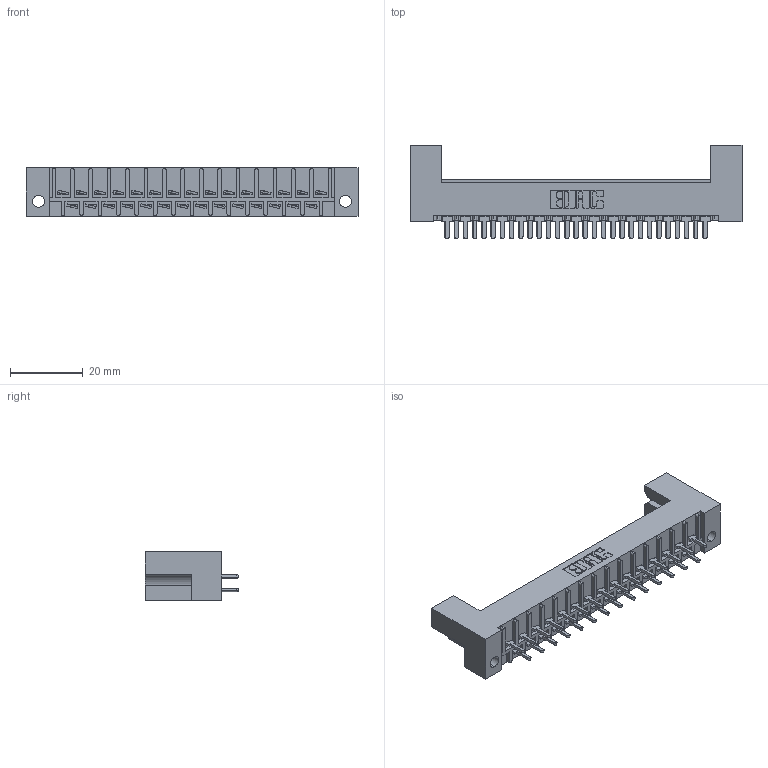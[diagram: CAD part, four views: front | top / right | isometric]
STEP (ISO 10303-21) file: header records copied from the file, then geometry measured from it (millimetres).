
FILE_DESCRIPTION (( 'STEP AP203' ), '1' );
FILE_NAME ('408-029-525-222.STEP', '2019-11-04T19:03:35', ( '' ), ( '' ), 'SwSTEP 2.0', 'SolidWorks 2016', '' );
FILE_SCHEMA (( 'CONFIG_CONTROL_DESIGN' ));
Length unit declared in the file: inch
Products named in the file (4): 408 Part_029 - 2; 408-029-525-222; 408-290-001_408-290-125 - Bottom; 408-290-001_408-290-125 - Top
Assembly tree (30 placements, depth 2):
  408-029-525-222
    408 Part_029 - 2
    408-290-001_408-290-125 - Bottom  x15
    408-290-001_408-290-125 - Top  x14
Bounding box: 91.59 x 25.73 x 13.49 mm (x, y, z)
Volume: 11652 mm3; surface area: 13282.5 mm2
Topology: 30 solids, 30 shells, 1737 faces, 4777 edges, 3106 vertices
Faces by surface type: plane 1307, cylinder 314, bspline 116
Entity records: 24727 total; most frequent: CARTESIAN_POINT 4311, ORIENTED_EDGE 4154, DIRECTION 3783, EDGE_CURVE 2077, LINE 1827, VECTOR 1827, VERTEX_POINT 1378, AXIS2_PLACEMENT_3D 978
